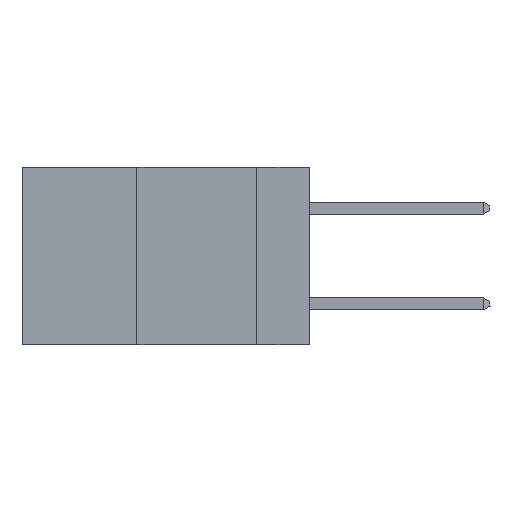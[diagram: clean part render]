
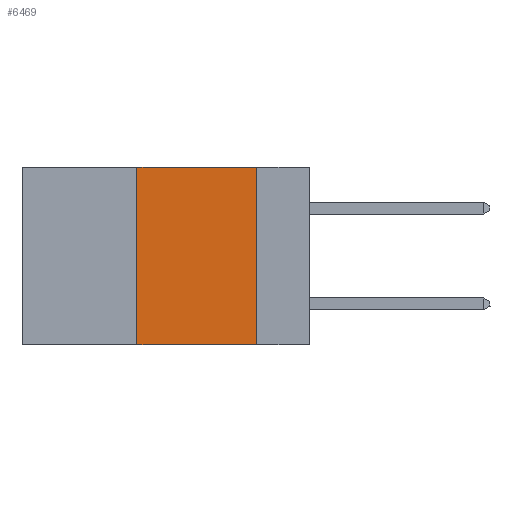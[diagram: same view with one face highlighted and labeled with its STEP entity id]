
A CAD part, left-side view. The second image highlights one B-rep face of the part: STEP entity #6469.
In plain terms, the highlighted planar face has unit normal (-1, 0, 0).
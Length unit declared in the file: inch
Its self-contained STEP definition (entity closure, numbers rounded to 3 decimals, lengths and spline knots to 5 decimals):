
#62 = VECTOR ( 'NONE', #15284, 39.37008 ) ;
#227 = VECTOR ( 'NONE', #11614, 39.37008 ) ;
#439 = DIRECTION ( 'NONE',  ( 0., 0., -1. ) ) ;
#1470 = ORIENTED_EDGE ( 'NONE', *, *, #17780, .F. ) ;
#1654 = DIRECTION ( 'NONE',  ( 1., 0., 0. ) ) ;
#2041 = VECTOR ( 'NONE', #14546, 39.37008 ) ;
#2414 = VECTOR ( 'NONE', #3679, 39.37008 ) ;
#3526 = CARTESIAN_POINT ( 'NONE',  ( 0., 0.11, -0.37 ) ) ;
#3679 = DIRECTION ( 'NONE',  ( 0., -1., 0. ) ) ;
#3764 = VERTEX_POINT ( 'NONE', #3526 ) ;
#3775 = LINE ( 'NONE', #5004, #2414 ) ;
#4253 = VERTEX_POINT ( 'NONE', #16695 ) ;
#5004 = CARTESIAN_POINT ( 'NONE',  ( 0., 0.6, 0. ) ) ;
#5025 = ORIENTED_EDGE ( 'NONE', *, *, #15425, .F. ) ;
#5870 = CARTESIAN_POINT ( 'NONE',  ( 0., 0.11, 0. ) ) ;
#6469 = ADVANCED_FACE ( 'NONE', ( #17394 ), #16084, .F. ) ;
#7288 = LINE ( 'NONE', #5870, #2041 ) ;
#8297 = VERTEX_POINT ( 'NONE', #8779 ) ;
#8779 = CARTESIAN_POINT ( 'NONE',  ( 0., 0.36, -0.37 ) ) ;
#9097 = EDGE_LOOP ( 'NONE', ( #9314, #5025, #1470, #17936 ) ) ;
#9125 = CARTESIAN_POINT ( 'NONE',  ( 0., 0.6, 0. ) ) ;
#9314 = ORIENTED_EDGE ( 'NONE', *, *, #13442, .F. ) ;
#9541 = CARTESIAN_POINT ( 'NONE',  ( 0., 0.36, 0. ) ) ;
#9742 = CARTESIAN_POINT ( 'NONE',  ( 0., 0.11, 0. ) ) ;
#11518 = LINE ( 'NONE', #15718, #227 ) ;
#11614 = DIRECTION ( 'NONE',  ( 0., -1., 0. ) ) ;
#12533 = EDGE_CURVE ( 'NONE', #8297, #3764, #11518, .T. ) ;
#13442 = EDGE_CURVE ( 'NONE', #13835, #3764, #7288, .T. ) ;
#13835 = VERTEX_POINT ( 'NONE', #9742 ) ;
#13972 = AXIS2_PLACEMENT_3D ( 'NONE', #9125, #1654, #439 ) ;
#14546 = DIRECTION ( 'NONE',  ( 0., 0., -1. ) ) ;
#15001 = LINE ( 'NONE', #9541, #62 ) ;
#15284 = DIRECTION ( 'NONE',  ( 0., 0., 1. ) ) ;
#15425 = EDGE_CURVE ( 'NONE', #4253, #13835, #3775, .T. ) ;
#15718 = CARTESIAN_POINT ( 'NONE',  ( 0., 0.6, -0.37 ) ) ;
#16084 = PLANE ( 'NONE',  #13972 ) ;
#16695 = CARTESIAN_POINT ( 'NONE',  ( 0., 0.36, 0. ) ) ;
#17394 = FACE_OUTER_BOUND ( 'NONE', #9097, .T. ) ;
#17780 = EDGE_CURVE ( 'NONE', #8297, #4253, #15001, .T. ) ;
#17936 = ORIENTED_EDGE ( 'NONE', *, *, #12533, .T. ) ;
